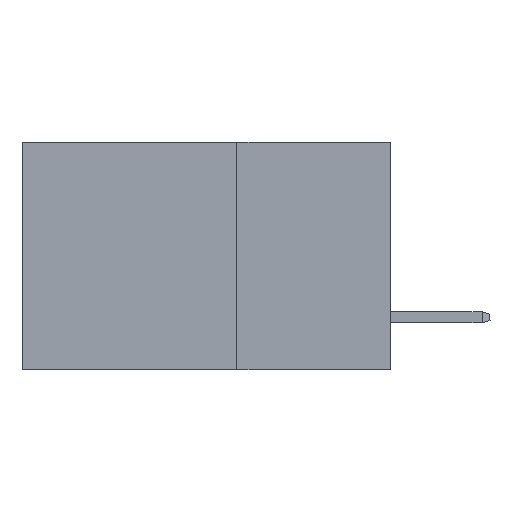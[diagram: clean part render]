
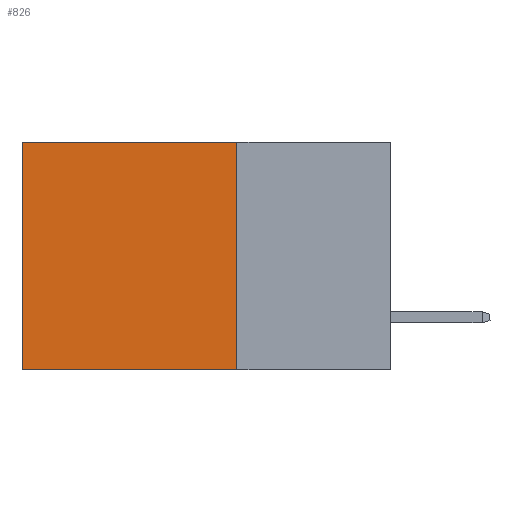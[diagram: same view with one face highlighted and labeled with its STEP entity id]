
A CAD part, left-side view. The second image highlights one B-rep face of the part: STEP entity #826.
In plain terms, the highlighted planar face has unit normal (-1, 0, 0).
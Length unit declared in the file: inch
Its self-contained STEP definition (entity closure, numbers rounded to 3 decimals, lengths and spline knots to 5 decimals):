
#71 = FACE_OUTER_BOUND ( 'NONE', #4972, .T. ) ;
#826 = ADVANCED_FACE ( 'NONE', ( #71 ), #2937, .F. ) ;
#903 = VERTEX_POINT ( 'NONE', #5629 ) ;
#1373 = VECTOR ( 'NONE', #9072, 39.37008 ) ;
#1446 = DIRECTION ( 'NONE',  ( 0., 1., 0. ) ) ;
#1475 = CARTESIAN_POINT ( 'NONE',  ( 0.2875, 0.25, -0.37 ) ) ;
#1501 = DIRECTION ( 'NONE',  ( 0., 0., -1. ) ) ;
#2021 = CARTESIAN_POINT ( 'NONE',  ( 0.2875, 0.25, 0. ) ) ;
#2053 = ORIENTED_EDGE ( 'NONE', *, *, #3986, .F. ) ;
#2117 = DIRECTION ( 'NONE',  ( 1., 0., 0. ) ) ;
#2797 = VERTEX_POINT ( 'NONE', #7848 ) ;
#2876 = LINE ( 'NONE', #7609, #8194 ) ;
#2890 = VECTOR ( 'NONE', #1446, 39.37008 ) ;
#2937 = PLANE ( 'NONE',  #5703 ) ;
#3240 = CARTESIAN_POINT ( 'NONE',  ( 0.2875, 0.6, -0.37 ) ) ;
#3320 = VECTOR ( 'NONE', #5624, 39.37008 ) ;
#3335 = EDGE_CURVE ( 'NONE', #2797, #4954, #9228, .T. ) ;
#3384 = VERTEX_POINT ( 'NONE', #5423 ) ;
#3905 = DIRECTION ( 'NONE',  ( 0., 0., -1. ) ) ;
#3986 = EDGE_CURVE ( 'NONE', #3384, #4954, #5081, .T. ) ;
#4281 = ORIENTED_EDGE ( 'NONE', *, *, #9764, .F. ) ;
#4954 = VERTEX_POINT ( 'NONE', #3240 ) ;
#4972 = EDGE_LOOP ( 'NONE', ( #7933, #2053, #4281, #8141 ) ) ;
#5081 = LINE ( 'NONE', #1475, #2890 ) ;
#5423 = CARTESIAN_POINT ( 'NONE',  ( 0.2875, 0.25, -0.37 ) ) ;
#5481 = LINE ( 'NONE', #9147, #1373 ) ;
#5624 = DIRECTION ( 'NONE',  ( 0., 0., -1. ) ) ;
#5629 = CARTESIAN_POINT ( 'NONE',  ( 0.2875, 0.25, 0. ) ) ;
#5646 = CARTESIAN_POINT ( 'NONE',  ( 0.2875, 0.6, 0. ) ) ;
#5703 = AXIS2_PLACEMENT_3D ( 'NONE', #2021, #2117, #1501 ) ;
#6968 = EDGE_CURVE ( 'NONE', #903, #2797, #5481, .T. ) ;
#7609 = CARTESIAN_POINT ( 'NONE',  ( 0.2875, 0.25, 0. ) ) ;
#7848 = CARTESIAN_POINT ( 'NONE',  ( 0.2875, 0.6, 0. ) ) ;
#7933 = ORIENTED_EDGE ( 'NONE', *, *, #3335, .T. ) ;
#8141 = ORIENTED_EDGE ( 'NONE', *, *, #6968, .T. ) ;
#8194 = VECTOR ( 'NONE', #3905, 39.37008 ) ;
#9072 = DIRECTION ( 'NONE',  ( 0., 1., 0. ) ) ;
#9147 = CARTESIAN_POINT ( 'NONE',  ( 0.2875, 0.25, 0. ) ) ;
#9228 = LINE ( 'NONE', #5646, #3320 ) ;
#9764 = EDGE_CURVE ( 'NONE', #903, #3384, #2876, .T. ) ;
